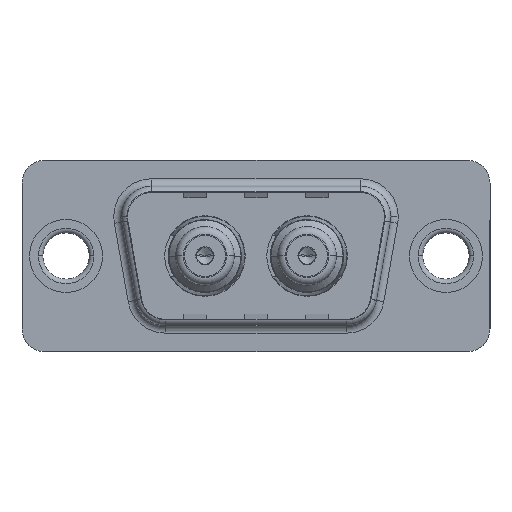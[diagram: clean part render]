
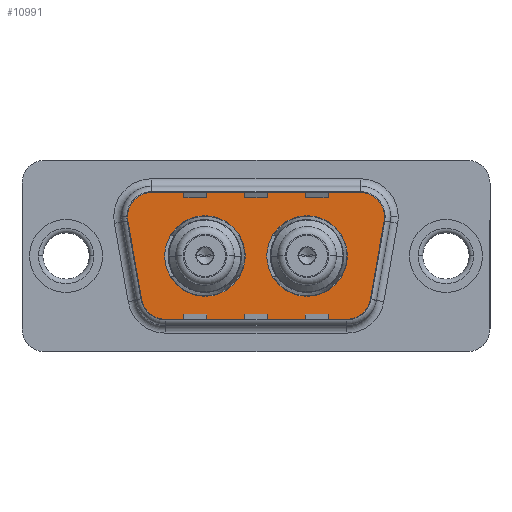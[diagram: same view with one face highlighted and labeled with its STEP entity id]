
A CAD part, top view. The second image highlights one B-rep face of the part: STEP entity #10991.
In plain terms, the highlighted planar face has unit normal (0, 0, 1).
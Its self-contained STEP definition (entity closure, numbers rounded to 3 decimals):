
#126 = EDGE_LOOP ( 'NONE', ( #9700, #1638 ) ) ;
#148 = CARTESIAN_POINT ( 'NONE',  ( 21.534, 2.553, 0. ) ) ;
#183 = ORIENTED_EDGE ( 'NONE', *, *, #10857, .T. ) ;
#244 = EDGE_CURVE ( 'NONE', #6271, #3192, #9150, .T. ) ;
#293 = DIRECTION ( 'NONE',  ( 0., 0., 1. ) ) ;
#324 = CARTESIAN_POINT ( 'NONE',  ( 13.21, 0., 0. ) ) ;
#333 = DIRECTION ( 'NONE',  ( -1., 0., 0. ) ) ;
#372 = CIRCLE ( 'NONE', #10314, 2. ) ;
#545 = FACE_OUTER_BOUND ( 'NONE', #6043, .T. ) ;
#694 = VERTEX_POINT ( 'NONE', #10052 ) ;
#771 = ORIENTED_EDGE ( 'NONE', *, *, #1847, .F. ) ;
#896 = AXIS2_PLACEMENT_3D ( 'NONE', #5429, #12075, #6375 ) ;
#923 = CIRCLE ( 'NONE', #4324, 2. ) ;
#997 = CARTESIAN_POINT ( 'NONE',  ( 5.436, 4.9, 0. ) ) ;
#1055 = DIRECTION ( 'NONE',  ( 1., 0., 0. ) ) ;
#1128 = DIRECTION ( 'NONE',  ( 0., 0., 1. ) ) ;
#1201 = CARTESIAN_POINT ( 'NONE',  ( 15.86, 0., 0. ) ) ;
#1323 = VERTEX_POINT ( 'NONE', #9892 ) ;
#1403 = EDGE_CURVE ( 'NONE', #7490, #7421, #7930, .T. ) ;
#1477 = CARTESIAN_POINT ( 'NONE',  ( 9.14, 0., 0. ) ) ;
#1638 = ORIENTED_EDGE ( 'NONE', *, *, #1403, .F. ) ;
#1731 = VECTOR ( 'NONE', #4279, 1000. ) ;
#1847 = EDGE_CURVE ( 'NONE', #3192, #6271, #6854, .T. ) ;
#2095 = CARTESIAN_POINT ( 'NONE',  ( 18.541, -2.9, 0. ) ) ;
#2119 = VERTEX_POINT ( 'NONE', #11073 ) ;
#2358 = LINE ( 'NONE', #5462, #12157 ) ;
#2370 = AXIS2_PLACEMENT_3D ( 'NONE', #4000, #293, #2954 ) ;
#2515 = EDGE_CURVE ( 'NONE', #1323, #4704, #923, .T. ) ;
#2524 = AXIS2_PLACEMENT_3D ( 'NONE', #4599, #11356, #3681 ) ;
#2954 = DIRECTION ( 'NONE',  ( -1., 0., 0. ) ) ;
#3036 = FACE_BOUND ( 'NONE', #126, .T. ) ;
#3057 = DIRECTION ( 'NONE',  ( 1., 0., 0. ) ) ;
#3171 = CARTESIAN_POINT ( 'NONE',  ( 6.459, -4.9, 0. ) ) ;
#3192 = VERTEX_POINT ( 'NONE', #3552 ) ;
#3212 = EDGE_CURVE ( 'NONE', #8937, #9337, #6677, .T. ) ;
#3417 = DIRECTION ( 'NONE',  ( 1., 0., 0. ) ) ;
#3480 = LINE ( 'NONE', #148, #8240 ) ;
#3552 = CARTESIAN_POINT ( 'NONE',  ( 11.79, 0., 0. ) ) ;
#3681 = DIRECTION ( 'NONE',  ( 1., 0., 0. ) ) ;
#3755 = ORIENTED_EDGE ( 'NONE', *, *, #11712, .T. ) ;
#3856 = CARTESIAN_POINT ( 'NONE',  ( 20.511, -3.247, 0. ) ) ;
#3986 = CARTESIAN_POINT ( 'NONE',  ( 4.489, -3.247, 0. ) ) ;
#4000 = CARTESIAN_POINT ( 'NONE',  ( 6.459, -2.9, 0. ) ) ;
#4123 = AXIS2_PLACEMENT_3D ( 'NONE', #7208, #9098, #3417 ) ;
#4133 = DIRECTION ( 'NONE',  ( 1., 0., 0. ) ) ;
#4205 = LINE ( 'NONE', #3171, #8965 ) ;
#4279 = DIRECTION ( 'NONE',  ( -1., 0., 0. ) ) ;
#4324 = AXIS2_PLACEMENT_3D ( 'NONE', #11671, #5961, #333 ) ;
#4392 = ORIENTED_EDGE ( 'NONE', *, *, #10680, .T. ) ;
#4407 = VERTEX_POINT ( 'NONE', #8174 ) ;
#4451 = CARTESIAN_POINT ( 'NONE',  ( 19.564, 4.9, 0. ) ) ;
#4599 = CARTESIAN_POINT ( 'NONE',  ( 9.14, 0., 0. ) ) ;
#4704 = VERTEX_POINT ( 'NONE', #4451 ) ;
#5161 = ORIENTED_EDGE ( 'NONE', *, *, #6251, .T. ) ;
#5359 = EDGE_CURVE ( 'NONE', #694, #8937, #2358, .T. ) ;
#5429 = CARTESIAN_POINT ( 'NONE',  ( 19.564, 2.9, 0. ) ) ;
#5462 = CARTESIAN_POINT ( 'NONE',  ( 3.466, 2.553, 0. ) ) ;
#5507 = AXIS2_PLACEMENT_3D ( 'NONE', #1201, #12009, #1055 ) ;
#5557 = DIRECTION ( 'NONE',  ( 1., 0., 0. ) ) ;
#5610 = DIRECTION ( 'NONE',  ( 0.174, -0.985, 0. ) ) ;
#5919 = EDGE_CURVE ( 'NONE', #7421, #7490, #9910, .T. ) ;
#5961 = DIRECTION ( 'NONE',  ( 0., 0., 1. ) ) ;
#6043 = EDGE_LOOP ( 'NONE', ( #6864, #4392, #3755, #12107, #9757, #5161, #7905, #8272, #183 ) ) ;
#6251 = EDGE_CURVE ( 'NONE', #10605, #694, #9454, .T. ) ;
#6271 = VERTEX_POINT ( 'NONE', #9649 ) ;
#6375 = DIRECTION ( 'NONE',  ( -1., 0., 0. ) ) ;
#6428 = CARTESIAN_POINT ( 'NONE',  ( 15.86, 0., 0. ) ) ;
#6677 = CIRCLE ( 'NONE', #2370, 2. ) ;
#6805 = CARTESIAN_POINT ( 'NONE',  ( 5.436, 2.9, 0. ) ) ;
#6854 = CIRCLE ( 'NONE', #2524, 2.65 ) ;
#6864 = ORIENTED_EDGE ( 'NONE', *, *, #8537, .T. ) ;
#7003 = ORIENTED_EDGE ( 'NONE', *, *, #244, .F. ) ;
#7155 = EDGE_CURVE ( 'NONE', #4704, #10605, #11223, .T. ) ;
#7208 = CARTESIAN_POINT ( 'NONE',  ( 18.541, -2.9, 0. ) ) ;
#7421 = VERTEX_POINT ( 'NONE', #10382 ) ;
#7490 = VERTEX_POINT ( 'NONE', #324 ) ;
#7748 = DIRECTION ( 'NONE',  ( 1., 0., 0. ) ) ;
#7788 = FACE_BOUND ( 'NONE', #10141, .T. ) ;
#7905 = ORIENTED_EDGE ( 'NONE', *, *, #5359, .T. ) ;
#7930 = CIRCLE ( 'NONE', #5507, 2.65 ) ;
#7958 = DIRECTION ( 'NONE',  ( 0., 0., 1. ) ) ;
#8060 = AXIS2_PLACEMENT_3D ( 'NONE', #6428, #7958, #5557 ) ;
#8174 = CARTESIAN_POINT ( 'NONE',  ( 21.534, 2.553, 0. ) ) ;
#8240 = VECTOR ( 'NONE', #8646, 1000. ) ;
#8272 = ORIENTED_EDGE ( 'NONE', *, *, #3212, .T. ) ;
#8473 = VERTEX_POINT ( 'NONE', #3856 ) ;
#8537 = EDGE_CURVE ( 'NONE', #2119, #8473, #372, .T. ) ;
#8646 = DIRECTION ( 'NONE',  ( 0.174, 0.985, 0. ) ) ;
#8732 = DIRECTION ( 'NONE',  ( 0., 0., 1. ) ) ;
#8937 = VERTEX_POINT ( 'NONE', #3986 ) ;
#8965 = VECTOR ( 'NONE', #10768, 1000. ) ;
#9098 = DIRECTION ( 'NONE',  ( 0., 0., 1. ) ) ;
#9150 = CIRCLE ( 'NONE', #11156, 2.65 ) ;
#9307 = CARTESIAN_POINT ( 'NONE',  ( 6.459, -4.9, 0. ) ) ;
#9337 = VERTEX_POINT ( 'NONE', #9307 ) ;
#9454 = CIRCLE ( 'NONE', #9726, 2. ) ;
#9649 = CARTESIAN_POINT ( 'NONE',  ( 6.49, 0., 0. ) ) ;
#9700 = ORIENTED_EDGE ( 'NONE', *, *, #5919, .F. ) ;
#9726 = AXIS2_PLACEMENT_3D ( 'NONE', #6805, #1128, #7748 ) ;
#9757 = ORIENTED_EDGE ( 'NONE', *, *, #7155, .T. ) ;
#9892 = CARTESIAN_POINT ( 'NONE',  ( 21.564, 2.9, 0. ) ) ;
#9910 = CIRCLE ( 'NONE', #8060, 2.65 ) ;
#10052 = CARTESIAN_POINT ( 'NONE',  ( 3.466, 2.553, 0. ) ) ;
#10141 = EDGE_LOOP ( 'NONE', ( #771, #7003 ) ) ;
#10314 = AXIS2_PLACEMENT_3D ( 'NONE', #2095, #8732, #3057 ) ;
#10382 = CARTESIAN_POINT ( 'NONE',  ( 18.51, 0., 0. ) ) ;
#10429 = CIRCLE ( 'NONE', #896, 2. ) ;
#10605 = VERTEX_POINT ( 'NONE', #997 ) ;
#10680 = EDGE_CURVE ( 'NONE', #8473, #4407, #3480, .T. ) ;
#10768 = DIRECTION ( 'NONE',  ( 1., 0., 0. ) ) ;
#10857 = EDGE_CURVE ( 'NONE', #9337, #2119, #4205, .T. ) ;
#10930 = CARTESIAN_POINT ( 'NONE',  ( 5.436, 4.9, 0. ) ) ;
#10956 = DIRECTION ( 'NONE',  ( 0., 0., 1. ) ) ;
#10978 = PLANE ( 'NONE',  #4123 ) ;
#10991 = ADVANCED_FACE ( 'NONE', ( #3036, #7788, #545 ), #10978, .T. ) ;
#11073 = CARTESIAN_POINT ( 'NONE',  ( 18.541, -4.9, 0. ) ) ;
#11156 = AXIS2_PLACEMENT_3D ( 'NONE', #1477, #10956, #4133 ) ;
#11223 = LINE ( 'NONE', #10930, #1731 ) ;
#11356 = DIRECTION ( 'NONE',  ( 0., 0., 1. ) ) ;
#11671 = CARTESIAN_POINT ( 'NONE',  ( 19.564, 2.9, 0. ) ) ;
#11712 = EDGE_CURVE ( 'NONE', #4407, #1323, #10429, .T. ) ;
#12009 = DIRECTION ( 'NONE',  ( 0., 0., 1. ) ) ;
#12075 = DIRECTION ( 'NONE',  ( 0., 0., 1. ) ) ;
#12107 = ORIENTED_EDGE ( 'NONE', *, *, #2515, .T. ) ;
#12157 = VECTOR ( 'NONE', #5610, 1000. ) ;
